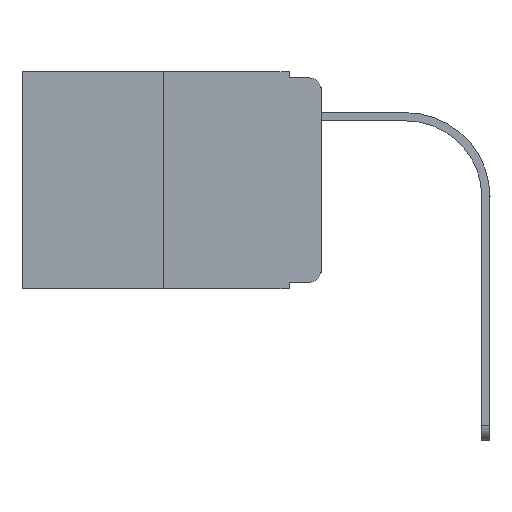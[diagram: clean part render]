
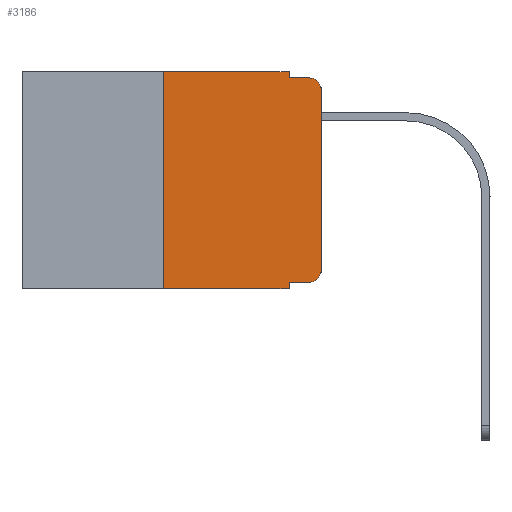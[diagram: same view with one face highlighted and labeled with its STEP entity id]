
A CAD part, left-side view. The second image highlights one B-rep face of the part: STEP entity #3186.
In plain terms, the highlighted planar face has unit normal (-1, 0, 0).
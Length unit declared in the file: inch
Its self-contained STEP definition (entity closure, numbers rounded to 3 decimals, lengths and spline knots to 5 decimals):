
#93 = CARTESIAN_POINT ( 'NONE',  ( 0., 0.02, -0.01 ) ) ;
#106 = EDGE_CURVE ( 'NONE', #5348, #9498, #5708, .T. ) ;
#254 = ORIENTED_EDGE ( 'NONE', *, *, #6499, .T. ) ;
#303 = VERTEX_POINT ( 'NONE', #14701 ) ;
#812 = CARTESIAN_POINT ( 'NONE',  ( 0., 0.25, 0. ) ) ;
#970 = CARTESIAN_POINT ( 'NONE',  ( 0., 0.02, -0.03 ) ) ;
#1389 = CARTESIAN_POINT ( 'NONE',  ( 0., 0.473, 0. ) ) ;
#1540 = AXIS2_PLACEMENT_3D ( 'NONE', #11963, #17665, #4855 ) ;
#1678 = ORIENTED_EDGE ( 'NONE', *, *, #13907, .F. ) ;
#1861 = PLANE ( 'NONE',  #1540 ) ;
#1924 = VERTEX_POINT ( 'NONE', #15779 ) ;
#2136 = EDGE_CURVE ( 'NONE', #5348, #7568, #3903, .T. ) ;
#2514 = ORIENTED_EDGE ( 'NONE', *, *, #15496, .F. ) ;
#2679 = CARTESIAN_POINT ( 'NONE',  ( 0., 0.051, -0.343 ) ) ;
#2792 = ORIENTED_EDGE ( 'NONE', *, *, #13312, .T. ) ;
#2976 = ORIENTED_EDGE ( 'NONE', *, *, #2136, .F. ) ;
#3186 = ADVANCED_FACE ( 'NONE', ( #17298 ), #1861, .F. ) ;
#3461 = CARTESIAN_POINT ( 'NONE',  ( 0., 0.051, 0. ) ) ;
#3628 = DIRECTION ( 'NONE',  ( 0., -1., 0. ) ) ;
#3686 = VECTOR ( 'NONE', #15578, 39.37008 ) ;
#3730 = DIRECTION ( 'NONE',  ( 0., 0., -1. ) ) ;
#3903 = LINE ( 'NONE', #4266, #3686 ) ;
#3962 = DIRECTION ( 'NONE',  ( 0., 0., -1. ) ) ;
#3980 = CARTESIAN_POINT ( 'NONE',  ( 0., 0., -0.03 ) ) ;
#4266 = CARTESIAN_POINT ( 'NONE',  ( 0., 0.25, 0. ) ) ;
#4452 = VECTOR ( 'NONE', #13475, 39.37008 ) ;
#4855 = DIRECTION ( 'NONE',  ( 0., 0., -1. ) ) ;
#5049 = CARTESIAN_POINT ( 'NONE',  ( 0., 0.051, 0. ) ) ;
#5348 = VERTEX_POINT ( 'NONE', #12398 ) ;
#5620 = AXIS2_PLACEMENT_3D ( 'NONE', #970, #12373, #3962 ) ;
#5623 = DIRECTION ( 'NONE',  ( 0., -1., 0. ) ) ;
#5708 = LINE ( 'NONE', #15436, #5974 ) ;
#5974 = VECTOR ( 'NONE', #5623, 39.37008 ) ;
#6348 = DIRECTION ( 'NONE',  ( 0., 0., 1. ) ) ;
#6470 = VERTEX_POINT ( 'NONE', #16243 ) ;
#6499 = EDGE_CURVE ( 'NONE', #6470, #10107, #12134, .T. ) ;
#7568 = VERTEX_POINT ( 'NONE', #812 ) ;
#7841 = CARTESIAN_POINT ( 'NONE',  ( 0., 0.051, -0.333 ) ) ;
#7878 = ORIENTED_EDGE ( 'NONE', *, *, #18387, .T. ) ;
#8113 = CARTESIAN_POINT ( 'NONE',  ( 0., 0.051, 0. ) ) ;
#8374 = ORIENTED_EDGE ( 'NONE', *, *, #12610, .T. ) ;
#8606 = LINE ( 'NONE', #1389, #14480 ) ;
#8917 = ORIENTED_EDGE ( 'NONE', *, *, #106, .T. ) ;
#9197 = VECTOR ( 'NONE', #6348, 39.37008 ) ;
#9408 = EDGE_LOOP ( 'NONE', ( #8374, #2792, #11482, #1678, #2514, #2976, #8917, #15045, #254, #7878 ) ) ;
#9498 = VERTEX_POINT ( 'NONE', #2679 ) ;
#10107 = VERTEX_POINT ( 'NONE', #16918 ) ;
#10714 = CIRCLE ( 'NONE', #11582, 0.02 ) ;
#10938 = VECTOR ( 'NONE', #15781, 39.37008 ) ;
#11482 = ORIENTED_EDGE ( 'NONE', *, *, #16198, .F. ) ;
#11582 = AXIS2_PLACEMENT_3D ( 'NONE', #14542, #14450, #13133 ) ;
#11920 = VECTOR ( 'NONE', #3628, 39.37008 ) ;
#11963 = CARTESIAN_POINT ( 'NONE',  ( 0., 0.473, 0. ) ) ;
#12083 = VERTEX_POINT ( 'NONE', #93 ) ;
#12134 = LINE ( 'NONE', #7841, #11920 ) ;
#12373 = DIRECTION ( 'NONE',  ( -1., 0., 0. ) ) ;
#12398 = CARTESIAN_POINT ( 'NONE',  ( 0., 0.25, -0.343 ) ) ;
#12610 = EDGE_CURVE ( 'NONE', #303, #15532, #17676, .T. ) ;
#12787 = EDGE_CURVE ( 'NONE', #6470, #9498, #13838, .T. ) ;
#13133 = DIRECTION ( 'NONE',  ( 0., 0., -1. ) ) ;
#13167 = LINE ( 'NONE', #14403, #10938 ) ;
#13312 = EDGE_CURVE ( 'NONE', #15532, #12083, #16991, .T. ) ;
#13475 = DIRECTION ( 'NONE',  ( 0., 0., -1. ) ) ;
#13838 = LINE ( 'NONE', #5049, #15746 ) ;
#13907 = EDGE_CURVE ( 'NONE', #18275, #1924, #16079, .T. ) ;
#14301 = DIRECTION ( 'NONE',  ( 0., -1., 0. ) ) ;
#14403 = CARTESIAN_POINT ( 'NONE',  ( 0., 0.051, -0.01 ) ) ;
#14450 = DIRECTION ( 'NONE',  ( -1., 0., 0. ) ) ;
#14480 = VECTOR ( 'NONE', #14301, 39.37008 ) ;
#14542 = CARTESIAN_POINT ( 'NONE',  ( 0., 0.02, -0.313 ) ) ;
#14701 = CARTESIAN_POINT ( 'NONE',  ( 0., 0., -0.313 ) ) ;
#15045 = ORIENTED_EDGE ( 'NONE', *, *, #12787, .F. ) ;
#15436 = CARTESIAN_POINT ( 'NONE',  ( 0., 0.473, -0.343 ) ) ;
#15496 = EDGE_CURVE ( 'NONE', #7568, #18275, #8606, .T. ) ;
#15532 = VERTEX_POINT ( 'NONE', #3980 ) ;
#15578 = DIRECTION ( 'NONE',  ( 0., 0., 1. ) ) ;
#15746 = VECTOR ( 'NONE', #3730, 39.37008 ) ;
#15779 = CARTESIAN_POINT ( 'NONE',  ( 0., 0.051, -0.01 ) ) ;
#15781 = DIRECTION ( 'NONE',  ( 0., -1., 0. ) ) ;
#16079 = LINE ( 'NONE', #3461, #4452 ) ;
#16198 = EDGE_CURVE ( 'NONE', #1924, #12083, #13167, .T. ) ;
#16243 = CARTESIAN_POINT ( 'NONE',  ( 0., 0.051, -0.333 ) ) ;
#16918 = CARTESIAN_POINT ( 'NONE',  ( 0., 0.02, -0.333 ) ) ;
#16991 = CIRCLE ( 'NONE', #5620, 0.02 ) ;
#17298 = FACE_OUTER_BOUND ( 'NONE', #9408, .T. ) ;
#17387 = CARTESIAN_POINT ( 'NONE',  ( 0., 0., 0. ) ) ;
#17665 = DIRECTION ( 'NONE',  ( 1., 0., 0. ) ) ;
#17676 = LINE ( 'NONE', #17387, #9197 ) ;
#18275 = VERTEX_POINT ( 'NONE', #8113 ) ;
#18387 = EDGE_CURVE ( 'NONE', #10107, #303, #10714, .T. ) ;
